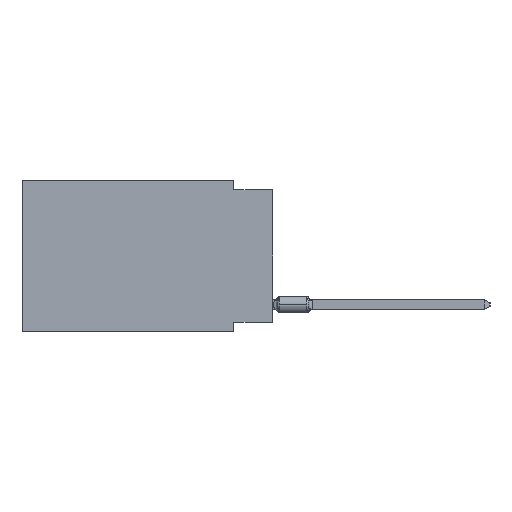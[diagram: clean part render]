
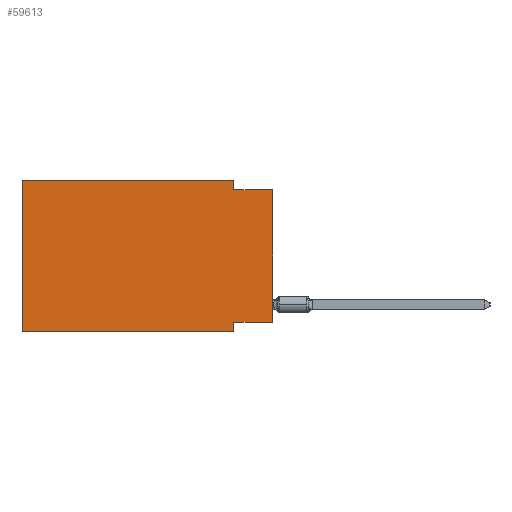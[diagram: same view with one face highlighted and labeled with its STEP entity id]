
A CAD part, left-side view. The second image highlights one B-rep face of the part: STEP entity #59613.
In plain terms, the highlighted planar face has unit normal (-1, 0, 0).
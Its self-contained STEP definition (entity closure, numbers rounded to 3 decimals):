
#3352 = LINE ( 'NONE', #56056, #38713 ) ;
#3957 = LINE ( 'NONE', #10011, #67262 ) ;
#4936 = CARTESIAN_POINT ( 'NONE',  ( 0., 16.383, -9.906 ) ) ;
#5046 = ORIENTED_EDGE ( 'NONE', *, *, #54899, .F. ) ;
#6268 = DIRECTION ( 'NONE',  ( 0., -1., 0. ) ) ;
#7731 = LINE ( 'NONE', #75061, #51245 ) ;
#8230 = LINE ( 'NONE', #22056, #66823 ) ;
#9721 = LINE ( 'NONE', #50724, #57401 ) ;
#10011 = CARTESIAN_POINT ( 'NONE',  ( 0., 16.383, 0. ) ) ;
#14445 = DIRECTION ( 'NONE',  ( 0., 0., -1. ) ) ;
#14970 = ORIENTED_EDGE ( 'NONE', *, *, #71931, .F. ) ;
#19387 = EDGE_CURVE ( 'NONE', #72299, #55492, #9721, .T. ) ;
#21574 = CARTESIAN_POINT ( 'NONE',  ( 0., 16.383, 0. ) ) ;
#22053 = CARTESIAN_POINT ( 'NONE',  ( 0., 16.383, 0. ) ) ;
#22056 = CARTESIAN_POINT ( 'NONE',  ( 0., 2.54, 0. ) ) ;
#22436 = EDGE_CURVE ( 'NONE', #78360, #55492, #29525, .T. ) ;
#23064 = CARTESIAN_POINT ( 'NONE',  ( 0., 2.54, -9.906 ) ) ;
#23104 = DIRECTION ( 'NONE',  ( 0., -1., 0. ) ) ;
#24066 = CARTESIAN_POINT ( 'NONE',  ( 0., 2.54, -9.906 ) ) ;
#25287 = CARTESIAN_POINT ( 'NONE',  ( 0., 0., -9.271 ) ) ;
#29525 = LINE ( 'NONE', #23064, #44669 ) ;
#30294 = DIRECTION ( 'NONE',  ( 0., 0., 1. ) ) ;
#33041 = VERTEX_POINT ( 'NONE', #82092 ) ;
#33812 = CARTESIAN_POINT ( 'NONE',  ( 0., 2.54, -9.271 ) ) ;
#34144 = LINE ( 'NONE', #22053, #56014 ) ;
#34278 = VERTEX_POINT ( 'NONE', #45639 ) ;
#36976 = LINE ( 'NONE', #73176, #38070 ) ;
#38070 = VECTOR ( 'NONE', #6268, 1000. ) ;
#38713 = VECTOR ( 'NONE', #82358, 1000. ) ;
#41842 = DIRECTION ( 'NONE',  ( 1., 0., 0. ) ) ;
#41843 = VERTEX_POINT ( 'NONE', #65046 ) ;
#42712 = PLANE ( 'NONE',  #82720 ) ;
#44669 = VECTOR ( 'NONE', #14445, 1000. ) ;
#45617 = EDGE_CURVE ( 'NONE', #72299, #83129, #3957, .T. ) ;
#45619 = EDGE_LOOP ( 'NONE', ( #54743, #51707, #14970, #5046, #74306, #52585, #59493, #78741 ) ) ;
#45639 = CARTESIAN_POINT ( 'NONE',  ( 0., 2.54, 0. ) ) ;
#46693 = DIRECTION ( 'NONE',  ( 0., 0., -1. ) ) ;
#47114 = DIRECTION ( 'NONE',  ( 0., -1., 0. ) ) ;
#50724 = CARTESIAN_POINT ( 'NONE',  ( 0., 16.383, -9.906 ) ) ;
#51245 = VECTOR ( 'NONE', #73783, 1000. ) ;
#51707 = ORIENTED_EDGE ( 'NONE', *, *, #52975, .F. ) ;
#52585 = ORIENTED_EDGE ( 'NONE', *, *, #19387, .T. ) ;
#52975 = EDGE_CURVE ( 'NONE', #33041, #41843, #36976, .T. ) ;
#54743 = ORIENTED_EDGE ( 'NONE', *, *, #82072, .T. ) ;
#54795 = CARTESIAN_POINT ( 'NONE',  ( 0., 16.383, 0. ) ) ;
#54899 = EDGE_CURVE ( 'NONE', #83129, #34278, #34144, .T. ) ;
#55492 = VERTEX_POINT ( 'NONE', #24066 ) ;
#56014 = VECTOR ( 'NONE', #47114, 1000. ) ;
#56056 = CARTESIAN_POINT ( 'NONE',  ( 0., 0., 0. ) ) ;
#57401 = VECTOR ( 'NONE', #23104, 1000. ) ;
#59493 = ORIENTED_EDGE ( 'NONE', *, *, #22436, .F. ) ;
#59613 = ADVANCED_FACE ( 'NONE', ( #60887 ), #42712, .F. ) ;
#60887 = FACE_OUTER_BOUND ( 'NONE', #45619, .T. ) ;
#61302 = DIRECTION ( 'NONE',  ( 0., 0., -1. ) ) ;
#62305 = EDGE_CURVE ( 'NONE', #84936, #78360, #7731, .T. ) ;
#65046 = CARTESIAN_POINT ( 'NONE',  ( 0., 0., -0.635 ) ) ;
#66823 = VECTOR ( 'NONE', #46693, 1000. ) ;
#67262 = VECTOR ( 'NONE', #30294, 1000. ) ;
#71931 = EDGE_CURVE ( 'NONE', #34278, #33041, #8230, .T. ) ;
#72299 = VERTEX_POINT ( 'NONE', #4936 ) ;
#73176 = CARTESIAN_POINT ( 'NONE',  ( 0., 0., -0.635 ) ) ;
#73783 = DIRECTION ( 'NONE',  ( 0., 1., 0. ) ) ;
#74306 = ORIENTED_EDGE ( 'NONE', *, *, #45617, .F. ) ;
#75061 = CARTESIAN_POINT ( 'NONE',  ( 0., 0., -9.271 ) ) ;
#78360 = VERTEX_POINT ( 'NONE', #33812 ) ;
#78741 = ORIENTED_EDGE ( 'NONE', *, *, #62305, .F. ) ;
#82072 = EDGE_CURVE ( 'NONE', #84936, #41843, #3352, .T. ) ;
#82092 = CARTESIAN_POINT ( 'NONE',  ( 0., 2.54, -0.635 ) ) ;
#82358 = DIRECTION ( 'NONE',  ( 0., 0., 1. ) ) ;
#82720 = AXIS2_PLACEMENT_3D ( 'NONE', #21574, #41842, #61302 ) ;
#83129 = VERTEX_POINT ( 'NONE', #54795 ) ;
#84936 = VERTEX_POINT ( 'NONE', #25287 ) ;
